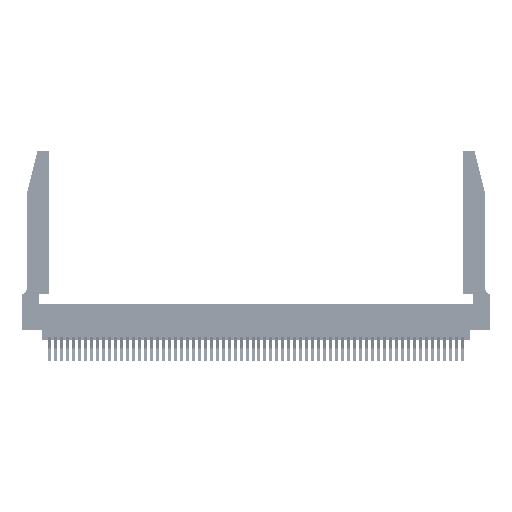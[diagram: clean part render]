
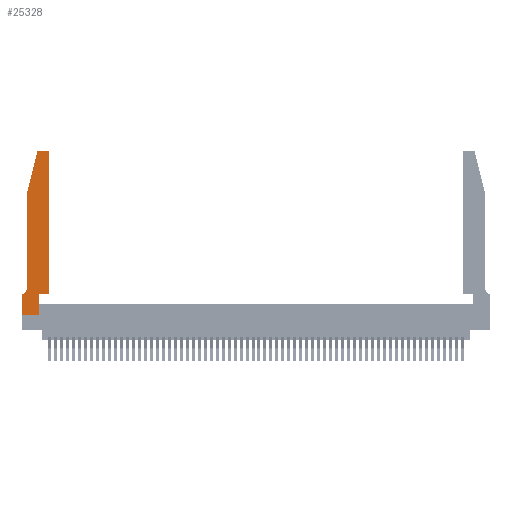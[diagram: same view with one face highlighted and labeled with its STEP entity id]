
A CAD part, top view. The second image highlights one B-rep face of the part: STEP entity #25328.
In plain terms, the highlighted planar face has unit normal (0, 0, 1).
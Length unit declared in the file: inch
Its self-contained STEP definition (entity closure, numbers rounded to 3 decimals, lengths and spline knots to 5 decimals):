
#162 = CARTESIAN_POINT ( 'NONE',  ( 0., 0.35, 0.37 ) ) ;
#1085 = EDGE_CURVE ( 'NONE', #52485, #44988, #25204, .T. ) ;
#1141 = CARTESIAN_POINT ( 'NONE',  ( 0.4505, 2.72, 0.37 ) ) ;
#1257 = CARTESIAN_POINT ( 'NONE',  ( 0.2605, 2.75, 0.37 ) ) ;
#2091 = ORIENTED_EDGE ( 'NONE', *, *, #29991, .T. ) ;
#2182 = DIRECTION ( 'NONE',  ( 0., 0., 1. ) ) ;
#2697 = DIRECTION ( 'NONE',  ( 0., 0., 1. ) ) ;
#3741 = VECTOR ( 'NONE', #50561, 39.37008 ) ;
#4185 = ORIENTED_EDGE ( 'NONE', *, *, #8125, .T. ) ;
#4324 = EDGE_CURVE ( 'NONE', #38581, #25448, #19432, .T. ) ;
#5716 = EDGE_LOOP ( 'NONE', ( #53865, #31068, #15387, #18652, #14549, #55057, #44329, #54362, #4185, #22022, #2091, #35569 ) ) ;
#6888 = CARTESIAN_POINT ( 'NONE',  ( 0., 0., 0.37 ) ) ;
#7239 = DIRECTION ( 'NONE',  ( 1., 0., 0. ) ) ;
#7445 = LINE ( 'NONE', #53210, #40788 ) ;
#8125 = EDGE_CURVE ( 'NONE', #25448, #56078, #7445, .T. ) ;
#8209 = CARTESIAN_POINT ( 'NONE',  ( 0.4205, 2.72, 0.37 ) ) ;
#8525 = CARTESIAN_POINT ( 'NONE',  ( 0.2865, 0.35, 0.37 ) ) ;
#10770 = CIRCLE ( 'NONE', #37562, 0.03 ) ;
#12204 = AXIS2_PLACEMENT_3D ( 'NONE', #28924, #2697, #33258 ) ;
#12625 = DIRECTION ( 'NONE',  ( 1., 0., 0. ) ) ;
#12626 = VECTOR ( 'NONE', #24409, 39.37008 ) ;
#12745 = VERTEX_POINT ( 'NONE', #42905 ) ;
#12798 = CARTESIAN_POINT ( 'NONE',  ( 0.284, 2.75, 0.37 ) ) ;
#13782 = VERTEX_POINT ( 'NONE', #41097 ) ;
#14549 = ORIENTED_EDGE ( 'NONE', *, *, #31966, .T. ) ;
#14927 = VECTOR ( 'NONE', #31864, 39.37008 ) ;
#15141 = FACE_OUTER_BOUND ( 'NONE', #5716, .T. ) ;
#15179 = EDGE_CURVE ( 'NONE', #26109, #38883, #47401, .T. ) ;
#15387 = ORIENTED_EDGE ( 'NONE', *, *, #37971, .T. ) ;
#16021 = CARTESIAN_POINT ( 'NONE',  ( 0.0755, 2., 0.37 ) ) ;
#17601 = VERTEX_POINT ( 'NONE', #1141 ) ;
#18652 = ORIENTED_EDGE ( 'NONE', *, *, #15179, .T. ) ;
#18691 = EDGE_CURVE ( 'NONE', #56078, #13782, #38566, .T. ) ;
#18711 = DIRECTION ( 'NONE',  ( 0., 1., 0. ) ) ;
#19432 = LINE ( 'NONE', #49922, #41119 ) ;
#19900 = VECTOR ( 'NONE', #44089, 39.37008 ) ;
#20152 = PLANE ( 'NONE',  #12204 ) ;
#20656 = CARTESIAN_POINT ( 'NONE',  ( 0.0755, 2., 0.37 ) ) ;
#20909 = CARTESIAN_POINT ( 'NONE',  ( 0.2865, 0., 0.37 ) ) ;
#21602 = AXIS2_PLACEMENT_3D ( 'NONE', #25723, #55757, #30099 ) ;
#22022 = ORIENTED_EDGE ( 'NONE', *, *, #18691, .T. ) ;
#22419 = EDGE_CURVE ( 'NONE', #27562, #36356, #23926, .T. ) ;
#23926 = LINE ( 'NONE', #52251, #46869 ) ;
#24233 = CARTESIAN_POINT ( 'NONE',  ( 0.0755, 2., 0.37 ) ) ;
#24409 = DIRECTION ( 'NONE',  ( 0., 1., 0. ) ) ;
#25204 = LINE ( 'NONE', #1257, #14927 ) ;
#25328 = ADVANCED_FACE ( 'NONE', ( #15141 ), #20152, .T. ) ;
#25448 = VERTEX_POINT ( 'NONE', #20909 ) ;
#25723 = CARTESIAN_POINT ( 'NONE',  ( 0.0055, 0.42, 0.37 ) ) ;
#26109 = VERTEX_POINT ( 'NONE', #20656 ) ;
#26227 = CARTESIAN_POINT ( 'NONE',  ( 0.0755, 0.42, 0.37 ) ) ;
#26534 = DIRECTION ( 'NONE',  ( -1., 0., 0. ) ) ;
#27562 = VERTEX_POINT ( 'NONE', #33061 ) ;
#28414 = CARTESIAN_POINT ( 'NONE',  ( 0.284, 2.72, 0.37 ) ) ;
#28924 = CARTESIAN_POINT ( 'NONE',  ( 0., 0.35, 0.37 ) ) ;
#29991 = EDGE_CURVE ( 'NONE', #13782, #17601, #45840, .T. ) ;
#30099 = DIRECTION ( 'NONE',  ( -1., 0., 0. ) ) ;
#31068 = ORIENTED_EDGE ( 'NONE', *, *, #50719, .T. ) ;
#31864 = DIRECTION ( 'NONE',  ( -1., 0., 0. ) ) ;
#31966 = EDGE_CURVE ( 'NONE', #38883, #27562, #46649, .T. ) ;
#32397 = CARTESIAN_POINT ( 'NONE',  ( 0.4205, 2.75, 0.37 ) ) ;
#32761 = DIRECTION ( 'NONE',  ( 1., 0., 0. ) ) ;
#33061 = CARTESIAN_POINT ( 'NONE',  ( 0.0055, 0.35, 0.37 ) ) ;
#33185 = AXIS2_PLACEMENT_3D ( 'NONE', #28414, #2182, #32761 ) ;
#33258 = DIRECTION ( 'NONE',  ( 1., 0., 0. ) ) ;
#35569 = ORIENTED_EDGE ( 'NONE', *, *, #52100, .T. ) ;
#36356 = VERTEX_POINT ( 'NONE', #162 ) ;
#37173 = LINE ( 'NONE', #16021, #3741 ) ;
#37562 = AXIS2_PLACEMENT_3D ( 'NONE', #8209, #38661, #12625 ) ;
#37931 = CARTESIAN_POINT ( 'NONE',  ( 0.4505, 0.35, 0.37 ) ) ;
#37971 = EDGE_CURVE ( 'NONE', #12745, #26109, #37173, .T. ) ;
#38566 = LINE ( 'NONE', #37931, #39900 ) ;
#38581 = VERTEX_POINT ( 'NONE', #6888 ) ;
#38661 = DIRECTION ( 'NONE',  ( 0., 0., 1. ) ) ;
#38883 = VERTEX_POINT ( 'NONE', #26227 ) ;
#39900 = VECTOR ( 'NONE', #7239, 39.37008 ) ;
#40788 = VECTOR ( 'NONE', #18711, 39.37008 ) ;
#41097 = CARTESIAN_POINT ( 'NONE',  ( 0.4505, 0.35, 0.37 ) ) ;
#41119 = VECTOR ( 'NONE', #45637, 39.37008 ) ;
#41423 = EDGE_CURVE ( 'NONE', #36356, #38581, #55605, .T. ) ;
#42905 = CARTESIAN_POINT ( 'NONE',  ( 0.25487, 2.72718, 0.37 ) ) ;
#44089 = DIRECTION ( 'NONE',  ( 0., -1., 0. ) ) ;
#44329 = ORIENTED_EDGE ( 'NONE', *, *, #41423, .T. ) ;
#44988 = VERTEX_POINT ( 'NONE', #12798 ) ;
#45637 = DIRECTION ( 'NONE',  ( 1., 0., 0. ) ) ;
#45840 = LINE ( 'NONE', #45887, #12626 ) ;
#45887 = CARTESIAN_POINT ( 'NONE',  ( 0.4505, 0.35, 0.37 ) ) ;
#46649 = CIRCLE ( 'NONE', #21602, 0.07 ) ;
#46869 = VECTOR ( 'NONE', #26534, 39.37008 ) ;
#47401 = LINE ( 'NONE', #24233, #48726 ) ;
#48214 = CARTESIAN_POINT ( 'NONE',  ( 0., 0., 0.37 ) ) ;
#48234 = CIRCLE ( 'NONE', #33185, 0.03 ) ;
#48726 = VECTOR ( 'NONE', #54291, 39.37008 ) ;
#49922 = CARTESIAN_POINT ( 'NONE',  ( 0., 0., 0.37 ) ) ;
#50561 = DIRECTION ( 'NONE',  ( -0.239, -0.971, 0. ) ) ;
#50719 = EDGE_CURVE ( 'NONE', #44988, #12745, #48234, .T. ) ;
#52100 = EDGE_CURVE ( 'NONE', #17601, #52485, #10770, .T. ) ;
#52251 = CARTESIAN_POINT ( 'NONE',  ( 0.0755, 0.35, 0.37 ) ) ;
#52485 = VERTEX_POINT ( 'NONE', #32397 ) ;
#53210 = CARTESIAN_POINT ( 'NONE',  ( 0.2865, 0.35, 0.37 ) ) ;
#53865 = ORIENTED_EDGE ( 'NONE', *, *, #1085, .T. ) ;
#54291 = DIRECTION ( 'NONE',  ( 0., -1., 0. ) ) ;
#54362 = ORIENTED_EDGE ( 'NONE', *, *, #4324, .T. ) ;
#55057 = ORIENTED_EDGE ( 'NONE', *, *, #22419, .T. ) ;
#55605 = LINE ( 'NONE', #48214, #19900 ) ;
#55757 = DIRECTION ( 'NONE',  ( 0., 0., -1. ) ) ;
#56078 = VERTEX_POINT ( 'NONE', #8525 ) ;
